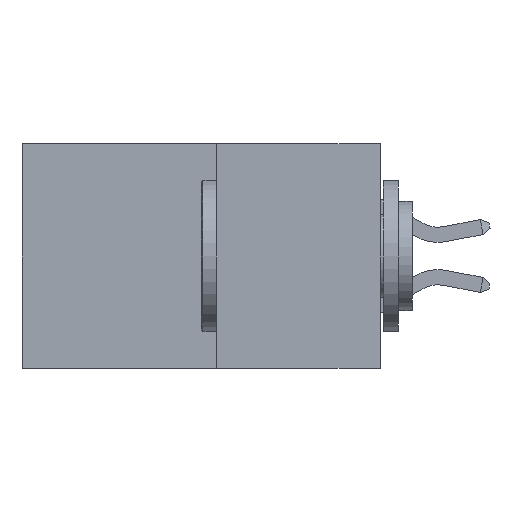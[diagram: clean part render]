
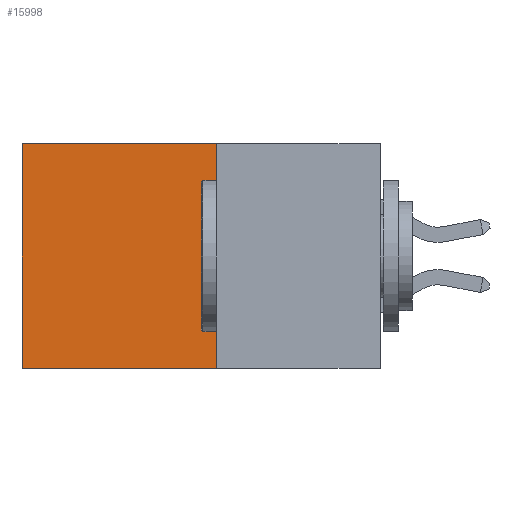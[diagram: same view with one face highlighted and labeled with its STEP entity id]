
A CAD part, left-side view. The second image highlights one B-rep face of the part: STEP entity #15998.
In plain terms, the highlighted planar face has unit normal (-1, 0, 0).
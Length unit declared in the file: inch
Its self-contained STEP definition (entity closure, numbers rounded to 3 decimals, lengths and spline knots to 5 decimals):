
#565 = DIRECTION ( 'NONE',  ( 0., 0., -1. ) ) ;
#3108 = CARTESIAN_POINT ( 'NONE',  ( 0.277, 0.27, -0.37 ) ) ;
#3967 = EDGE_CURVE ( 'NONE', #6266, #24583, #18025, .T. ) ;
#4566 = VECTOR ( 'NONE', #4812, 39.37008 ) ;
#4812 = DIRECTION ( 'NONE',  ( 0., 0., -1. ) ) ;
#5062 = CARTESIAN_POINT ( 'NONE',  ( 0.277, 0.27, -0.37 ) ) ;
#6266 = VERTEX_POINT ( 'NONE', #20895 ) ;
#6796 = VECTOR ( 'NONE', #20616, 39.37008 ) ;
#9165 = DIRECTION ( 'NONE',  ( 0., 1., 0. ) ) ;
#9509 = EDGE_LOOP ( 'NONE', ( #19370, #20722, #28330, #16108 ) ) ;
#9592 = VERTEX_POINT ( 'NONE', #31530 ) ;
#10684 = CARTESIAN_POINT ( 'NONE',  ( 0.277, 0.27, -0.37 ) ) ;
#11614 = VERTEX_POINT ( 'NONE', #24161 ) ;
#11886 = VECTOR ( 'NONE', #9165, 39.37008 ) ;
#12300 = EDGE_CURVE ( 'NONE', #6266, #11614, #18566, .T. ) ;
#13338 = DIRECTION ( 'NONE',  ( 0., 1., 0. ) ) ;
#14346 = LINE ( 'NONE', #18149, #6796 ) ;
#15321 = EDGE_CURVE ( 'NONE', #24583, #9592, #16851, .T. ) ;
#15789 = DIRECTION ( 'NONE',  ( 1., 0., 0. ) ) ;
#15998 = ADVANCED_FACE ( 'NONE', ( #17194 ), #23119, .F. ) ;
#16108 = ORIENTED_EDGE ( 'NONE', *, *, #12300, .T. ) ;
#16691 = CARTESIAN_POINT ( 'NONE',  ( 0.277, 0.27, 0. ) ) ;
#16851 = LINE ( 'NONE', #30684, #30779 ) ;
#17194 = FACE_OUTER_BOUND ( 'NONE', #9509, .T. ) ;
#18025 = LINE ( 'NONE', #5062, #4566 ) ;
#18149 = CARTESIAN_POINT ( 'NONE',  ( 0.277, 0.59, -0.37 ) ) ;
#18566 = LINE ( 'NONE', #16691, #11886 ) ;
#18639 = EDGE_CURVE ( 'NONE', #11614, #9592, #14346, .T. ) ;
#19370 = ORIENTED_EDGE ( 'NONE', *, *, #18639, .T. ) ;
#20616 = DIRECTION ( 'NONE',  ( 0., 0., -1. ) ) ;
#20722 = ORIENTED_EDGE ( 'NONE', *, *, #15321, .F. ) ;
#20895 = CARTESIAN_POINT ( 'NONE',  ( 0.277, 0.27, 0. ) ) ;
#23119 = PLANE ( 'NONE',  #23895 ) ;
#23895 = AXIS2_PLACEMENT_3D ( 'NONE', #10684, #15789, #565 ) ;
#24161 = CARTESIAN_POINT ( 'NONE',  ( 0.277, 0.59, 0. ) ) ;
#24583 = VERTEX_POINT ( 'NONE', #3108 ) ;
#28330 = ORIENTED_EDGE ( 'NONE', *, *, #3967, .F. ) ;
#30684 = CARTESIAN_POINT ( 'NONE',  ( 0.277, 0.27, -0.37 ) ) ;
#30779 = VECTOR ( 'NONE', #13338, 39.37008 ) ;
#31530 = CARTESIAN_POINT ( 'NONE',  ( 0.277, 0.59, -0.37 ) ) ;
